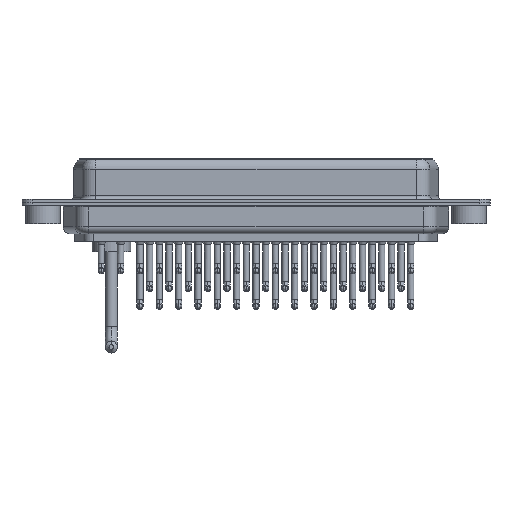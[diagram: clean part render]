
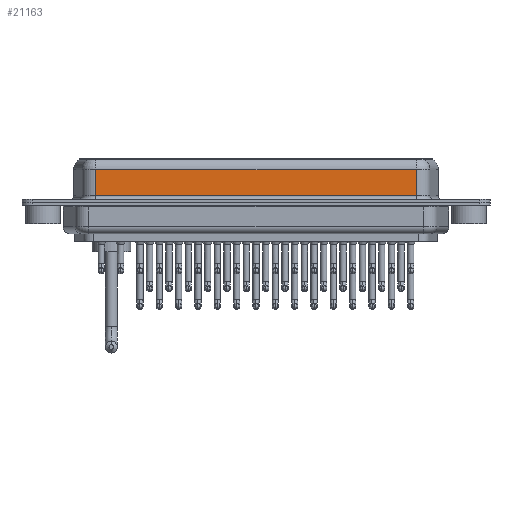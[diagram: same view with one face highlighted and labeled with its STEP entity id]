
A CAD part, front view. The second image highlights one B-rep face of the part: STEP entity #21163.
In plain terms, the highlighted planar face has unit normal (0, -1, 0).
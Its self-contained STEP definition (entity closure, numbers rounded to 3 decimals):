
#483 = PLANE ( 'NONE',  #29700 ) ;
#1404 = CARTESIAN_POINT ( 'NONE',  ( 7.59, -5.375, 6.4 ) ) ;
#3395 = VECTOR ( 'NONE', #21686, 1000. ) ;
#3441 = LINE ( 'NONE', #16522, #3395 ) ;
#3570 = VECTOR ( 'NONE', #31440, 1000. ) ;
#5840 = FACE_OUTER_BOUND ( 'NONE', #21846, .T. ) ;
#6358 = VERTEX_POINT ( 'NONE', #22015 ) ;
#6738 = EDGE_CURVE ( 'NONE', #6358, #22910, #23892, .T. ) ;
#8397 = VERTEX_POINT ( 'NONE', #10400 ) ;
#10400 = CARTESIAN_POINT ( 'NONE',  ( 53.41, -5.375, 0.9 ) ) ;
#11017 = DIRECTION ( 'NONE',  ( 0., 1., 0. ) ) ;
#13448 = ORIENTED_EDGE ( 'NONE', *, *, #23413, .T. ) ;
#13895 = ORIENTED_EDGE ( 'NONE', *, *, #19950, .F. ) ;
#15276 = ORIENTED_EDGE ( 'NONE', *, *, #6738, .T. ) ;
#15347 = VECTOR ( 'NONE', #28280, 1000. ) ;
#15989 = DIRECTION ( 'NONE',  ( 0., 0., 1. ) ) ;
#16522 = CARTESIAN_POINT ( 'NONE',  ( 53.41, -5.375, 0.9 ) ) ;
#17792 = LINE ( 'NONE', #30182, #15347 ) ;
#18346 = VERTEX_POINT ( 'NONE', #29338 ) ;
#19161 = LINE ( 'NONE', #1404, #29863 ) ;
#19950 = EDGE_CURVE ( 'NONE', #6358, #8397, #17792, .T. ) ;
#21163 = ADVANCED_FACE ( 'NONE', ( #5840 ), #483, .F. ) ;
#21686 = DIRECTION ( 'NONE',  ( 1., 0., 0. ) ) ;
#21846 = EDGE_LOOP ( 'NONE', ( #13895, #15276, #29968, #13448 ) ) ;
#22015 = CARTESIAN_POINT ( 'NONE',  ( 53.41, -5.375, 4.65 ) ) ;
#22910 = VERTEX_POINT ( 'NONE', #31590 ) ;
#23413 = EDGE_CURVE ( 'NONE', #18346, #8397, #3441, .T. ) ;
#23551 = CARTESIAN_POINT ( 'NONE',  ( 53.41, -5.375, 4.65 ) ) ;
#23892 = LINE ( 'NONE', #23551, #3570 ) ;
#27236 = DIRECTION ( 'NONE',  ( 0., 0., -1. ) ) ;
#28280 = DIRECTION ( 'NONE',  ( 0., 0., -1. ) ) ;
#29338 = CARTESIAN_POINT ( 'NONE',  ( 7.59, -5.375, 0.9 ) ) ;
#29700 = AXIS2_PLACEMENT_3D ( 'NONE', #32146, #11017, #15989 ) ;
#29863 = VECTOR ( 'NONE', #27236, 1000. ) ;
#29968 = ORIENTED_EDGE ( 'NONE', *, *, #30223, .T. ) ;
#30182 = CARTESIAN_POINT ( 'NONE',  ( 53.41, -5.375, 6.4 ) ) ;
#30223 = EDGE_CURVE ( 'NONE', #22910, #18346, #19161, .T. ) ;
#31440 = DIRECTION ( 'NONE',  ( -1., 0., 0. ) ) ;
#31590 = CARTESIAN_POINT ( 'NONE',  ( 7.59, -5.375, 4.65 ) ) ;
#32146 = CARTESIAN_POINT ( 'NONE',  ( 53.41, -5.375, 6.4 ) ) ;
